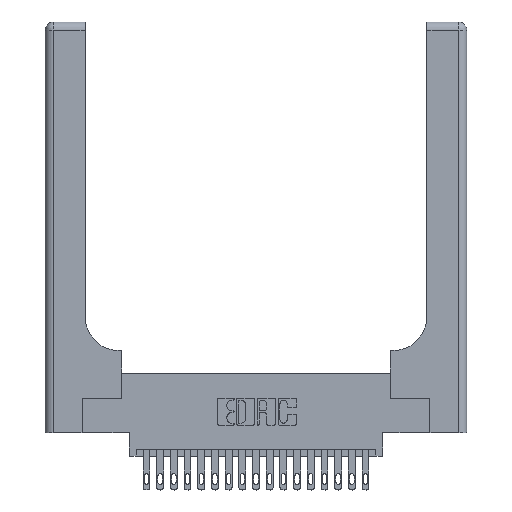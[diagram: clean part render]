
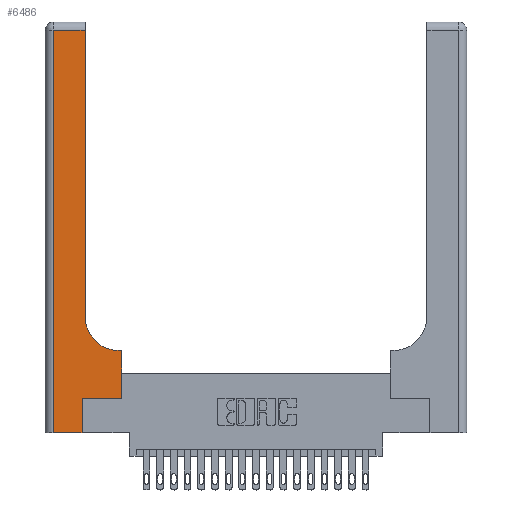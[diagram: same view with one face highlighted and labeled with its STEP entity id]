
A CAD part, top view. The second image highlights one B-rep face of the part: STEP entity #6486.
In plain terms, the highlighted planar face has unit normal (0, 0, 1).
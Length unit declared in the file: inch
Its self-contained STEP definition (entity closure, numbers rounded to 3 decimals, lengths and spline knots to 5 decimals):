
#320 = DIRECTION ( 'NONE',  ( 1., 0., 0. ) ) ;
#432 = LINE ( 'NONE', #14010, #17396 ) ;
#458 = CARTESIAN_POINT ( 'NONE',  ( 0.269, 0.25, 0.37 ) ) ;
#826 = AXIS2_PLACEMENT_3D ( 'NONE', #11707, #6692, #10156 ) ;
#1471 = LINE ( 'NONE', #9054, #5436 ) ;
#1961 = VERTEX_POINT ( 'NONE', #17771 ) ;
#2065 = ORIENTED_EDGE ( 'NONE', *, *, #19803, .T. ) ;
#2428 = CARTESIAN_POINT ( 'NONE',  ( 0.2915, 0.85, 0.37 ) ) ;
#2734 = DIRECTION ( 'NONE',  ( 0., 0., -1. ) ) ;
#3137 = LINE ( 'NONE', #8616, #3933 ) ;
#3824 = LINE ( 'NONE', #7059, #12551 ) ;
#3870 = EDGE_CURVE ( 'NONE', #1961, #4360, #3824, .T. ) ;
#3933 = VECTOR ( 'NONE', #11825, 39.37008 ) ;
#4094 = EDGE_CURVE ( 'NONE', #4360, #8747, #5637, .T. ) ;
#4360 = VERTEX_POINT ( 'NONE', #12841 ) ;
#4451 = CARTESIAN_POINT ( 'NONE',  ( 0.269, 0., 0.37 ) ) ;
#4672 = AXIS2_PLACEMENT_3D ( 'NONE', #7849, #2734, #7767 ) ;
#4679 = LINE ( 'NONE', #18828, #16630 ) ;
#4693 = CARTESIAN_POINT ( 'NONE',  ( 0.2915, 0.6, 0.37 ) ) ;
#5436 = VECTOR ( 'NONE', #14894, 39.37008 ) ;
#5476 = CARTESIAN_POINT ( 'NONE',  ( 0.06, 3., 0.37 ) ) ;
#5637 = LINE ( 'NONE', #4693, #14415 ) ;
#5639 = EDGE_CURVE ( 'NONE', #15327, #7236, #16206, .T. ) ;
#5659 = DIRECTION ( 'NONE',  ( 0., 1., 0. ) ) ;
#6187 = CARTESIAN_POINT ( 'NONE',  ( 0.5415, 0.6, 0.37 ) ) ;
#6486 = ADVANCED_FACE ( 'NONE', ( #18304 ), #13453, .F. ) ;
#6692 = DIRECTION ( 'NONE',  ( 0., 0., -1. ) ) ;
#7059 = CARTESIAN_POINT ( 'NONE',  ( 0.5585, 0.25, 0.37 ) ) ;
#7148 = VECTOR ( 'NONE', #9811, 39.37008 ) ;
#7236 = VERTEX_POINT ( 'NONE', #9091 ) ;
#7767 = DIRECTION ( 'NONE',  ( 1., 0., 0. ) ) ;
#7784 = EDGE_CURVE ( 'NONE', #16444, #17366, #4679, .T. ) ;
#7849 = CARTESIAN_POINT ( 'NONE',  ( 0.5415, 0.85, 0.37 ) ) ;
#8385 = EDGE_CURVE ( 'NONE', #17366, #1961, #432, .T. ) ;
#8616 = CARTESIAN_POINT ( 'NONE',  ( 0.2915, 3., 0.37 ) ) ;
#8747 = VERTEX_POINT ( 'NONE', #6187 ) ;
#9054 = CARTESIAN_POINT ( 'NONE',  ( 0., 2.94, 0.37 ) ) ;
#9091 = CARTESIAN_POINT ( 'NONE',  ( 0.06, 0., 0.37 ) ) ;
#9258 = EDGE_CURVE ( 'NONE', #9403, #15327, #1471, .T. ) ;
#9403 = VERTEX_POINT ( 'NONE', #19602 ) ;
#9811 = DIRECTION ( 'NONE',  ( 0., -1., 0. ) ) ;
#9861 = CIRCLE ( 'NONE', #4672, 0.25 ) ;
#10156 = DIRECTION ( 'NONE',  ( -1., 0., 0. ) ) ;
#10417 = ORIENTED_EDGE ( 'NONE', *, *, #7784, .T. ) ;
#11222 = ORIENTED_EDGE ( 'NONE', *, *, #5639, .T. ) ;
#11675 = DIRECTION ( 'NONE',  ( -1., 0., 0. ) ) ;
#11707 = CARTESIAN_POINT ( 'NONE',  ( 0., 3., 0.37 ) ) ;
#11825 = DIRECTION ( 'NONE',  ( 0., 1., 0. ) ) ;
#12501 = DIRECTION ( 'NONE',  ( 1., 0., 0. ) ) ;
#12551 = VECTOR ( 'NONE', #5659, 39.37008 ) ;
#12565 = CARTESIAN_POINT ( 'NONE',  ( 0., 0., 0.37 ) ) ;
#12841 = CARTESIAN_POINT ( 'NONE',  ( 0.5585, 0.6, 0.37 ) ) ;
#13158 = VERTEX_POINT ( 'NONE', #2428 ) ;
#13453 = PLANE ( 'NONE',  #826 ) ;
#13536 = ORIENTED_EDGE ( 'NONE', *, *, #8385, .T. ) ;
#14010 = CARTESIAN_POINT ( 'NONE',  ( 0.269, 0.25, 0.37 ) ) ;
#14415 = VECTOR ( 'NONE', #11675, 39.37008 ) ;
#14539 = LINE ( 'NONE', #12565, #18547 ) ;
#14894 = DIRECTION ( 'NONE',  ( -1., 0., 0. ) ) ;
#15327 = VERTEX_POINT ( 'NONE', #19490 ) ;
#15853 = ORIENTED_EDGE ( 'NONE', *, *, #17571, .T. ) ;
#16206 = LINE ( 'NONE', #5476, #7148 ) ;
#16444 = VERTEX_POINT ( 'NONE', #4451 ) ;
#16575 = ORIENTED_EDGE ( 'NONE', *, *, #4094, .T. ) ;
#16630 = VECTOR ( 'NONE', #20347, 39.37008 ) ;
#17301 = ORIENTED_EDGE ( 'NONE', *, *, #9258, .T. ) ;
#17366 = VERTEX_POINT ( 'NONE', #458 ) ;
#17396 = VECTOR ( 'NONE', #320, 39.37008 ) ;
#17529 = EDGE_LOOP ( 'NONE', ( #21024, #17301, #11222, #2065, #10417, #13536, #20941, #16575, #15853 ) ) ;
#17571 = EDGE_CURVE ( 'NONE', #8747, #13158, #9861, .T. ) ;
#17771 = CARTESIAN_POINT ( 'NONE',  ( 0.5585, 0.25, 0.37 ) ) ;
#18304 = FACE_OUTER_BOUND ( 'NONE', #17529, .T. ) ;
#18547 = VECTOR ( 'NONE', #12501, 39.37008 ) ;
#18828 = CARTESIAN_POINT ( 'NONE',  ( 0.269, 0., 0.37 ) ) ;
#19490 = CARTESIAN_POINT ( 'NONE',  ( 0.06, 2.94, 0.37 ) ) ;
#19602 = CARTESIAN_POINT ( 'NONE',  ( 0.2915, 2.94, 0.37 ) ) ;
#19803 = EDGE_CURVE ( 'NONE', #7236, #16444, #14539, .T. ) ;
#20347 = DIRECTION ( 'NONE',  ( 0., 1., 0. ) ) ;
#20814 = EDGE_CURVE ( 'NONE', #13158, #9403, #3137, .T. ) ;
#20941 = ORIENTED_EDGE ( 'NONE', *, *, #3870, .T. ) ;
#21024 = ORIENTED_EDGE ( 'NONE', *, *, #20814, .T. ) ;
